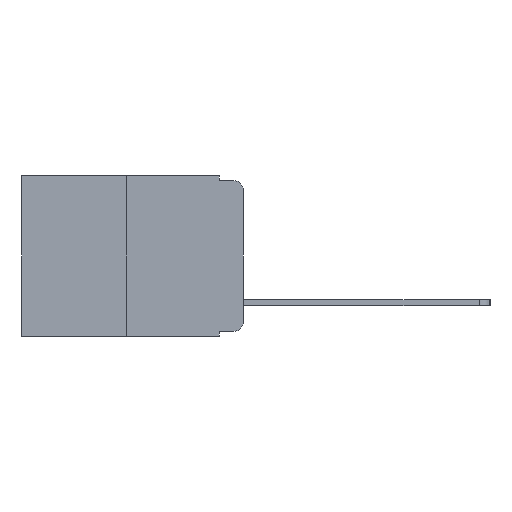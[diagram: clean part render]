
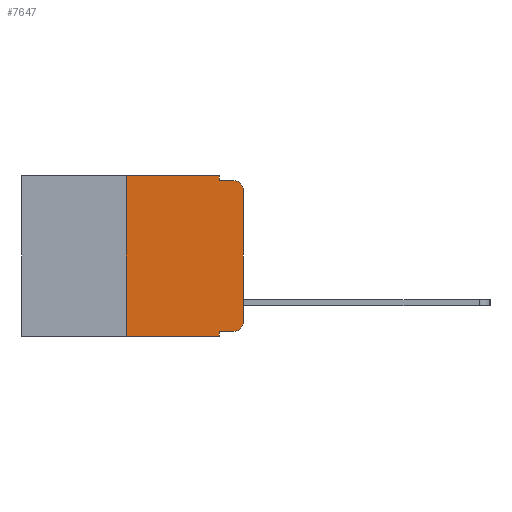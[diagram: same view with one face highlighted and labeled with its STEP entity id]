
A CAD part, left-side view. The second image highlights one B-rep face of the part: STEP entity #7647.
In plain terms, the highlighted planar face has unit normal (-1, 0, 0).
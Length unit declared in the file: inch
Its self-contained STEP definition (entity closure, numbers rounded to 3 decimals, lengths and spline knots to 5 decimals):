
#20 = AXIS2_PLACEMENT_3D ( 'NONE', #13924, #7334, #14995 ) ;
#26 = LINE ( 'NONE', #14306, #8832 ) ;
#209 = CIRCLE ( 'NONE', #4906, 0.02 ) ;
#226 = DIRECTION ( 'NONE',  ( 0., 0., -1. ) ) ;
#375 = VERTEX_POINT ( 'NONE', #12897 ) ;
#422 = EDGE_CURVE ( 'NONE', #1797, #2522, #432, .T. ) ;
#432 = LINE ( 'NONE', #12249, #9113 ) ;
#620 = EDGE_CURVE ( 'NONE', #2264, #7310, #7912, .T. ) ;
#722 = VECTOR ( 'NONE', #8816, 39.37008 ) ;
#839 = VECTOR ( 'NONE', #1283, 39.37008 ) ;
#1283 = DIRECTION ( 'NONE',  ( 0., 0., 1. ) ) ;
#1387 = EDGE_CURVE ( 'NONE', #1797, #12314, #8221, .T. ) ;
#1797 = VERTEX_POINT ( 'NONE', #13366 ) ;
#1856 = DIRECTION ( 'NONE',  ( 0., 0., -1. ) ) ;
#1877 = ORIENTED_EDGE ( 'NONE', *, *, #4005, .T. ) ;
#1896 = AXIS2_PLACEMENT_3D ( 'NONE', #12343, #9064, #1856 ) ;
#2264 = VERTEX_POINT ( 'NONE', #14628 ) ;
#2311 = EDGE_CURVE ( 'NONE', #8842, #2264, #8734, .T. ) ;
#2522 = VERTEX_POINT ( 'NONE', #4267 ) ;
#2609 = DIRECTION ( 'NONE',  ( -1., 0., 0. ) ) ;
#2670 = CARTESIAN_POINT ( 'NONE',  ( 0., 0., -0.03 ) ) ;
#2717 = ORIENTED_EDGE ( 'NONE', *, *, #14854, .T. ) ;
#2847 = ORIENTED_EDGE ( 'NONE', *, *, #4881, .F. ) ;
#3264 = DIRECTION ( 'NONE',  ( 0., 0., 1. ) ) ;
#4005 = EDGE_CURVE ( 'NONE', #8842, #12314, #7624, .T. ) ;
#4077 = EDGE_CURVE ( 'NONE', #7310, #14088, #26, .T. ) ;
#4267 = CARTESIAN_POINT ( 'NONE',  ( 0., 0.02, -0.333 ) ) ;
#4293 = LINE ( 'NONE', #9872, #722 ) ;
#4628 = CARTESIAN_POINT ( 'NONE',  ( 0., 0.02, -0.01 ) ) ;
#4881 = EDGE_CURVE ( 'NONE', #14088, #12436, #4293, .T. ) ;
#4901 = ORIENTED_EDGE ( 'NONE', *, *, #2311, .F. ) ;
#4906 = AXIS2_PLACEMENT_3D ( 'NONE', #9663, #2609, #10793 ) ;
#5276 = CARTESIAN_POINT ( 'NONE',  ( 0., 0.051, 0. ) ) ;
#5478 = DIRECTION ( 'NONE',  ( 0., -1., 0. ) ) ;
#5668 = EDGE_CURVE ( 'NONE', #15001, #12436, #209, .T. ) ;
#6100 = CARTESIAN_POINT ( 'NONE',  ( 0., 0.473, 0. ) ) ;
#6171 = ORIENTED_EDGE ( 'NONE', *, *, #6469, .T. ) ;
#6469 = EDGE_CURVE ( 'NONE', #375, #15001, #7880, .T. ) ;
#6713 = EDGE_LOOP ( 'NONE', ( #6171, #9189, #2847, #6921, #9873, #4901, #1877, #14159, #8681, #2717 ) ) ;
#6921 = ORIENTED_EDGE ( 'NONE', *, *, #4077, .F. ) ;
#7310 = VERTEX_POINT ( 'NONE', #5276 ) ;
#7334 = DIRECTION ( 'NONE',  ( -1., 0., 0. ) ) ;
#7467 = CARTESIAN_POINT ( 'NONE',  ( 0., 0., 0. ) ) ;
#7533 = VECTOR ( 'NONE', #13504, 39.37008 ) ;
#7624 = LINE ( 'NONE', #12026, #13145 ) ;
#7647 = ADVANCED_FACE ( 'NONE', ( #8206 ), #7971, .F. ) ;
#7847 = CARTESIAN_POINT ( 'NONE',  ( 0., 0.051, 0. ) ) ;
#7880 = LINE ( 'NONE', #7467, #839 ) ;
#7912 = LINE ( 'NONE', #6100, #7533 ) ;
#7971 = PLANE ( 'NONE',  #1896 ) ;
#8206 = FACE_OUTER_BOUND ( 'NONE', #6713, .T. ) ;
#8221 = LINE ( 'NONE', #7847, #13677 ) ;
#8408 = VECTOR ( 'NONE', #3264, 39.37008 ) ;
#8553 = CARTESIAN_POINT ( 'NONE',  ( 0., 0.051, -0.01 ) ) ;
#8681 = ORIENTED_EDGE ( 'NONE', *, *, #422, .T. ) ;
#8734 = LINE ( 'NONE', #9840, #8408 ) ;
#8816 = DIRECTION ( 'NONE',  ( 0., -1., 0. ) ) ;
#8832 = VECTOR ( 'NONE', #9952, 39.37008 ) ;
#8842 = VERTEX_POINT ( 'NONE', #14703 ) ;
#9064 = DIRECTION ( 'NONE',  ( 1., 0., 0. ) ) ;
#9096 = CARTESIAN_POINT ( 'NONE',  ( 0., 0.051, -0.343 ) ) ;
#9113 = VECTOR ( 'NONE', #5478, 39.37008 ) ;
#9189 = ORIENTED_EDGE ( 'NONE', *, *, #5668, .T. ) ;
#9663 = CARTESIAN_POINT ( 'NONE',  ( 0., 0.02, -0.03 ) ) ;
#9840 = CARTESIAN_POINT ( 'NONE',  ( 0., 0.25, 0. ) ) ;
#9872 = CARTESIAN_POINT ( 'NONE',  ( 0., 0.051, -0.01 ) ) ;
#9873 = ORIENTED_EDGE ( 'NONE', *, *, #620, .F. ) ;
#9952 = DIRECTION ( 'NONE',  ( 0., 0., -1. ) ) ;
#10793 = DIRECTION ( 'NONE',  ( 0., 0., -1. ) ) ;
#10804 = CIRCLE ( 'NONE', #20, 0.02 ) ;
#12026 = CARTESIAN_POINT ( 'NONE',  ( 0., 0.473, -0.343 ) ) ;
#12249 = CARTESIAN_POINT ( 'NONE',  ( 0., 0.051, -0.333 ) ) ;
#12314 = VERTEX_POINT ( 'NONE', #9096 ) ;
#12343 = CARTESIAN_POINT ( 'NONE',  ( 0., 0.473, 0. ) ) ;
#12436 = VERTEX_POINT ( 'NONE', #4628 ) ;
#12897 = CARTESIAN_POINT ( 'NONE',  ( 0., 0., -0.313 ) ) ;
#13132 = DIRECTION ( 'NONE',  ( 0., -1., 0. ) ) ;
#13145 = VECTOR ( 'NONE', #13132, 39.37008 ) ;
#13366 = CARTESIAN_POINT ( 'NONE',  ( 0., 0.051, -0.333 ) ) ;
#13504 = DIRECTION ( 'NONE',  ( 0., -1., 0. ) ) ;
#13677 = VECTOR ( 'NONE', #226, 39.37008 ) ;
#13924 = CARTESIAN_POINT ( 'NONE',  ( 0., 0.02, -0.313 ) ) ;
#14088 = VERTEX_POINT ( 'NONE', #8553 ) ;
#14159 = ORIENTED_EDGE ( 'NONE', *, *, #1387, .F. ) ;
#14306 = CARTESIAN_POINT ( 'NONE',  ( 0., 0.051, 0. ) ) ;
#14628 = CARTESIAN_POINT ( 'NONE',  ( 0., 0.25, 0. ) ) ;
#14703 = CARTESIAN_POINT ( 'NONE',  ( 0., 0.25, -0.343 ) ) ;
#14854 = EDGE_CURVE ( 'NONE', #2522, #375, #10804, .T. ) ;
#14995 = DIRECTION ( 'NONE',  ( 0., 0., -1. ) ) ;
#15001 = VERTEX_POINT ( 'NONE', #2670 ) ;
